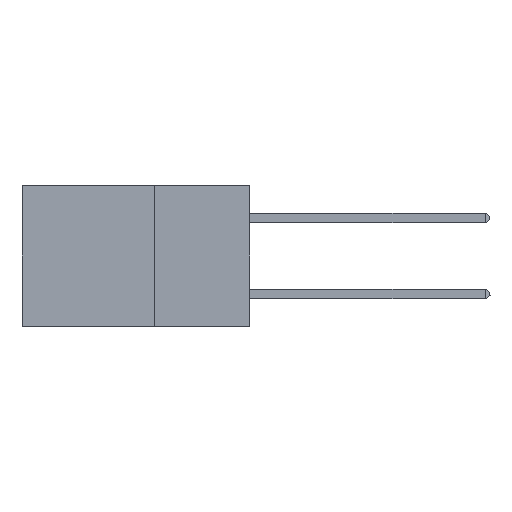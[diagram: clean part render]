
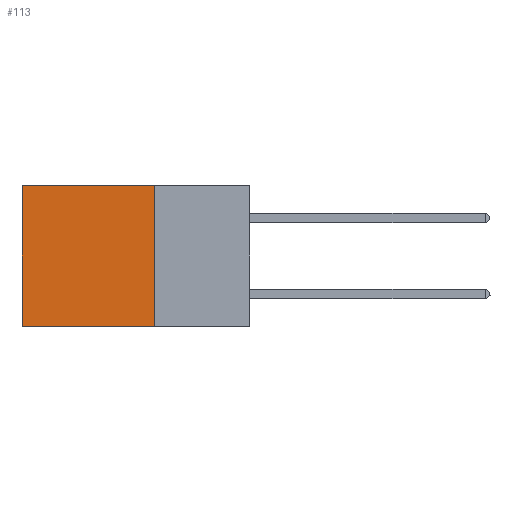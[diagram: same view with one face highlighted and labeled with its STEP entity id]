
A CAD part, left-side view. The second image highlights one B-rep face of the part: STEP entity #113.
In plain terms, the highlighted planar face has unit normal (-1, 0, 0).
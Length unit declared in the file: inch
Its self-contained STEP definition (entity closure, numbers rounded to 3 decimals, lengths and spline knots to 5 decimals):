
#113 = ADVANCED_FACE ( 'NONE', ( #13693 ), #18432, .F. ) ;
#605 = VERTEX_POINT ( 'NONE', #20718 ) ;
#953 = DIRECTION ( 'NONE',  ( 0., 1., 0. ) ) ;
#1140 = DIRECTION ( 'NONE',  ( 0., 1., 0. ) ) ;
#3229 = LINE ( 'NONE', #24867, #3922 ) ;
#3574 = DIRECTION ( 'NONE',  ( 0., 0., -1. ) ) ;
#3922 = VECTOR ( 'NONE', #953, 39.37008 ) ;
#4039 = DIRECTION ( 'NONE',  ( 0., 0., -1. ) ) ;
#5039 = VECTOR ( 'NONE', #4039, 39.37008 ) ;
#7775 = CARTESIAN_POINT ( 'NONE',  ( 0.2875, 0.25, 0. ) ) ;
#9113 = AXIS2_PLACEMENT_3D ( 'NONE', #9377, #20936, #12259 ) ;
#9240 = EDGE_CURVE ( 'NONE', #13231, #605, #3229, .T. ) ;
#9377 = CARTESIAN_POINT ( 'NONE',  ( 0.2875, 0.25, 0. ) ) ;
#9384 = CARTESIAN_POINT ( 'NONE',  ( 0.2875, 0.6, 0. ) ) ;
#9828 = ORIENTED_EDGE ( 'NONE', *, *, #25602, .F. ) ;
#9889 = EDGE_CURVE ( 'NONE', #10270, #605, #17364, .T. ) ;
#10012 = CARTESIAN_POINT ( 'NONE',  ( 0.2875, 0.25, 0. ) ) ;
#10270 = VERTEX_POINT ( 'NONE', #9384 ) ;
#10292 = ORIENTED_EDGE ( 'NONE', *, *, #9889, .T. ) ;
#12184 = EDGE_CURVE ( 'NONE', #26129, #10270, #18205, .T. ) ;
#12259 = DIRECTION ( 'NONE',  ( 0., 0., -1. ) ) ;
#12536 = CARTESIAN_POINT ( 'NONE',  ( 0.2875, 0.25, 0. ) ) ;
#13231 = VERTEX_POINT ( 'NONE', #14877 ) ;
#13693 = FACE_OUTER_BOUND ( 'NONE', #27602, .T. ) ;
#14078 = ORIENTED_EDGE ( 'NONE', *, *, #9240, .F. ) ;
#14877 = CARTESIAN_POINT ( 'NONE',  ( 0.2875, 0.25, -0.37 ) ) ;
#17246 = CARTESIAN_POINT ( 'NONE',  ( 0.2875, 0.6, 0. ) ) ;
#17348 = VECTOR ( 'NONE', #3574, 39.37008 ) ;
#17364 = LINE ( 'NONE', #17246, #5039 ) ;
#18205 = LINE ( 'NONE', #7775, #26071 ) ;
#18432 = PLANE ( 'NONE',  #9113 ) ;
#20718 = CARTESIAN_POINT ( 'NONE',  ( 0.2875, 0.6, -0.37 ) ) ;
#20936 = DIRECTION ( 'NONE',  ( 1., 0., 0. ) ) ;
#23171 = LINE ( 'NONE', #10012, #17348 ) ;
#24867 = CARTESIAN_POINT ( 'NONE',  ( 0.2875, 0.25, -0.37 ) ) ;
#25602 = EDGE_CURVE ( 'NONE', #26129, #13231, #23171, .T. ) ;
#26071 = VECTOR ( 'NONE', #1140, 39.37008 ) ;
#26129 = VERTEX_POINT ( 'NONE', #12536 ) ;
#27213 = ORIENTED_EDGE ( 'NONE', *, *, #12184, .T. ) ;
#27602 = EDGE_LOOP ( 'NONE', ( #10292, #14078, #9828, #27213 ) ) ;
